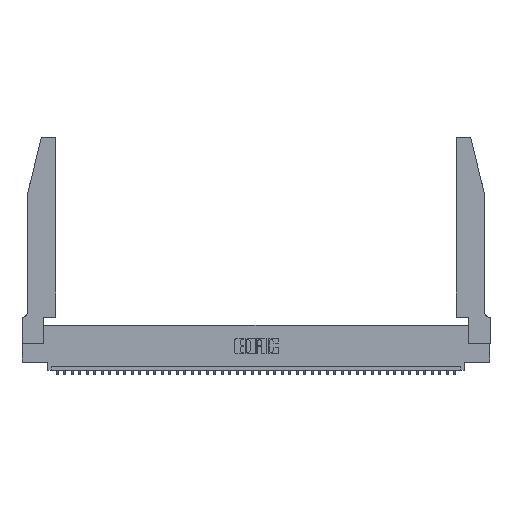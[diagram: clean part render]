
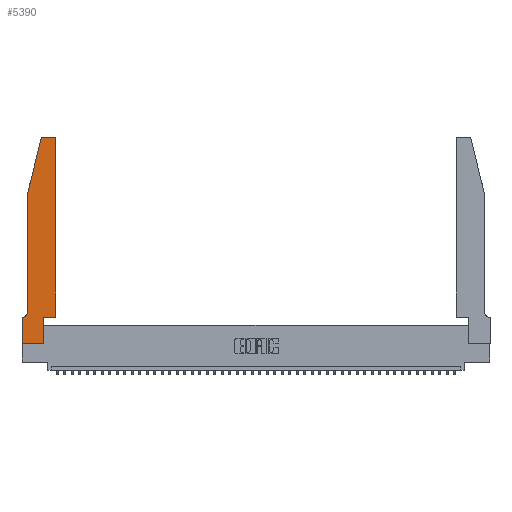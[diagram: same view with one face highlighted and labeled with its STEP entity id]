
A CAD part, top view. The second image highlights one B-rep face of the part: STEP entity #5390.
In plain terms, the highlighted planar face has unit normal (0, 0, 1).
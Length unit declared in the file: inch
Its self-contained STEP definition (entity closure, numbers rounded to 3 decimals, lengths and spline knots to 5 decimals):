
#191 = DIRECTION ( 'NONE',  ( 0., 1., 0. ) ) ;
#806 = VECTOR ( 'NONE', #6028, 39.37008 ) ;
#989 = CARTESIAN_POINT ( 'NONE',  ( 0.2865, 0.35, 0.37 ) ) ;
#1644 = VERTEX_POINT ( 'NONE', #21481 ) ;
#1873 = CARTESIAN_POINT ( 'NONE',  ( 0.0755, 0.42, 0.37 ) ) ;
#1937 = LINE ( 'NONE', #42458, #41774 ) ;
#2378 = ORIENTED_EDGE ( 'NONE', *, *, #20064, .T. ) ;
#2583 = AXIS2_PLACEMENT_3D ( 'NONE', #17825, #21153, #38533 ) ;
#2833 = ORIENTED_EDGE ( 'NONE', *, *, #18375, .T. ) ;
#2907 = EDGE_CURVE ( 'NONE', #39275, #1644, #37408, .T. ) ;
#3115 = LINE ( 'NONE', #5863, #16230 ) ;
#3315 = CARTESIAN_POINT ( 'NONE',  ( 0.2865, 0.35, 0.37 ) ) ;
#3512 = DIRECTION ( 'NONE',  ( 1., 0., 0. ) ) ;
#4232 = AXIS2_PLACEMENT_3D ( 'NONE', #39001, #29052, #32171 ) ;
#4340 = EDGE_CURVE ( 'NONE', #42796, #12998, #38647, .T. ) ;
#4575 = DIRECTION ( 'NONE',  ( 1., 0., 0. ) ) ;
#4819 = ORIENTED_EDGE ( 'NONE', *, *, #34659, .T. ) ;
#5390 = ADVANCED_FACE ( 'NONE', ( #12595 ), #5482, .T. ) ;
#5440 = CARTESIAN_POINT ( 'NONE',  ( 0.4505, 2.72, 0.37 ) ) ;
#5482 = PLANE ( 'NONE',  #21039 ) ;
#5863 = CARTESIAN_POINT ( 'NONE',  ( 0.0755, 2., 0.37 ) ) ;
#6028 = DIRECTION ( 'NONE',  ( 1., 0., 0. ) ) ;
#7231 = VERTEX_POINT ( 'NONE', #1873 ) ;
#7233 = EDGE_LOOP ( 'NONE', ( #24595, #9767, #9809, #29688, #2378, #16241, #39439, #4819, #2833, #15806, #39345, #33789 ) ) ;
#7916 = VERTEX_POINT ( 'NONE', #989 ) ;
#9767 = ORIENTED_EDGE ( 'NONE', *, *, #2907, .T. ) ;
#9809 = ORIENTED_EDGE ( 'NONE', *, *, #25964, .T. ) ;
#10091 = EDGE_CURVE ( 'NONE', #30700, #7231, #3115, .T. ) ;
#11860 = CARTESIAN_POINT ( 'NONE',  ( 0.2605, 2.75, 0.37 ) ) ;
#12595 = FACE_OUTER_BOUND ( 'NONE', #7233, .T. ) ;
#12653 = EDGE_CURVE ( 'NONE', #7916, #32591, #25085, .T. ) ;
#12816 = CIRCLE ( 'NONE', #2583, 0.07 ) ;
#12870 = CARTESIAN_POINT ( 'NONE',  ( 0.4505, 0.35, 0.37 ) ) ;
#12997 = CARTESIAN_POINT ( 'NONE',  ( 0., 0., 0.37 ) ) ;
#12998 = VERTEX_POINT ( 'NONE', #36776 ) ;
#14085 = CARTESIAN_POINT ( 'NONE',  ( 0.0755, 2., 0.37 ) ) ;
#14971 = CARTESIAN_POINT ( 'NONE',  ( 0.4505, 0.35, 0.37 ) ) ;
#15395 = AXIS2_PLACEMENT_3D ( 'NONE', #34845, #24881, #4575 ) ;
#15483 = DIRECTION ( 'NONE',  ( 0., -1., 0. ) ) ;
#15806 = ORIENTED_EDGE ( 'NONE', *, *, #12653, .T. ) ;
#15988 = CARTESIAN_POINT ( 'NONE',  ( 0.0755, 0.35, 0.37 ) ) ;
#16230 = VECTOR ( 'NONE', #26606, 39.37008 ) ;
#16241 = ORIENTED_EDGE ( 'NONE', *, *, #38518, .T. ) ;
#16411 = EDGE_CURVE ( 'NONE', #32591, #42796, #41674, .T. ) ;
#17486 = DIRECTION ( 'NONE',  ( -0.239, -0.971, 0. ) ) ;
#17825 = CARTESIAN_POINT ( 'NONE',  ( 0.0055, 0.42, 0.37 ) ) ;
#18375 = EDGE_CURVE ( 'NONE', #20291, #7916, #23511, .T. ) ;
#19219 = DIRECTION ( 'NONE',  ( -1., 0., 0. ) ) ;
#20064 = EDGE_CURVE ( 'NONE', #7231, #38523, #12816, .T. ) ;
#20291 = VERTEX_POINT ( 'NONE', #29174 ) ;
#20858 = VERTEX_POINT ( 'NONE', #12997 ) ;
#21039 = AXIS2_PLACEMENT_3D ( 'NONE', #33361, #30671, #3512 ) ;
#21153 = DIRECTION ( 'NONE',  ( 0., 0., -1. ) ) ;
#21481 = CARTESIAN_POINT ( 'NONE',  ( 0.25487, 2.72718, 0.37 ) ) ;
#23511 = LINE ( 'NONE', #3315, #27242 ) ;
#24120 = VECTOR ( 'NONE', #42094, 39.37008 ) ;
#24223 = CARTESIAN_POINT ( 'NONE',  ( 0.0755, 2., 0.37 ) ) ;
#24317 = VECTOR ( 'NONE', #17486, 39.37008 ) ;
#24595 = ORIENTED_EDGE ( 'NONE', *, *, #30277, .T. ) ;
#24881 = DIRECTION ( 'NONE',  ( 0., 0., 1. ) ) ;
#25085 = LINE ( 'NONE', #31417, #36790 ) ;
#25964 = EDGE_CURVE ( 'NONE', #1644, #30700, #37609, .T. ) ;
#26606 = DIRECTION ( 'NONE',  ( 0., -1., 0. ) ) ;
#26845 = VERTEX_POINT ( 'NONE', #39020 ) ;
#26910 = EDGE_CURVE ( 'NONE', #26845, #20858, #1937, .T. ) ;
#27242 = VECTOR ( 'NONE', #191, 39.37008 ) ;
#29052 = DIRECTION ( 'NONE',  ( 0., 0., 1. ) ) ;
#29174 = CARTESIAN_POINT ( 'NONE',  ( 0.2865, 0., 0.37 ) ) ;
#29439 = CARTESIAN_POINT ( 'NONE',  ( 0., 0., 0.37 ) ) ;
#29449 = CARTESIAN_POINT ( 'NONE',  ( 0.0055, 0.35, 0.37 ) ) ;
#29688 = ORIENTED_EDGE ( 'NONE', *, *, #10091, .T. ) ;
#29821 = VECTOR ( 'NONE', #19219, 39.37008 ) ;
#30277 = EDGE_CURVE ( 'NONE', #12998, #39275, #42588, .T. ) ;
#30671 = DIRECTION ( 'NONE',  ( 0., 0., 1. ) ) ;
#30700 = VERTEX_POINT ( 'NONE', #24223 ) ;
#31417 = CARTESIAN_POINT ( 'NONE',  ( 0.4505, 0.35, 0.37 ) ) ;
#32171 = DIRECTION ( 'NONE',  ( 1., 0., 0. ) ) ;
#32535 = VECTOR ( 'NONE', #39118, 39.37008 ) ;
#32591 = VERTEX_POINT ( 'NONE', #12870 ) ;
#33361 = CARTESIAN_POINT ( 'NONE',  ( 0., 0.35, 0.37 ) ) ;
#33789 = ORIENTED_EDGE ( 'NONE', *, *, #4340, .T. ) ;
#34286 = CARTESIAN_POINT ( 'NONE',  ( 0.284, 2.75, 0.37 ) ) ;
#34659 = EDGE_CURVE ( 'NONE', #20858, #20291, #42230, .T. ) ;
#34845 = CARTESIAN_POINT ( 'NONE',  ( 0.4205, 2.72, 0.37 ) ) ;
#35641 = LINE ( 'NONE', #15988, #29821 ) ;
#36776 = CARTESIAN_POINT ( 'NONE',  ( 0.4205, 2.75, 0.37 ) ) ;
#36790 = VECTOR ( 'NONE', #41830, 39.37008 ) ;
#37408 = CIRCLE ( 'NONE', #4232, 0.03 ) ;
#37609 = LINE ( 'NONE', #14085, #24317 ) ;
#38518 = EDGE_CURVE ( 'NONE', #38523, #26845, #35641, .T. ) ;
#38523 = VERTEX_POINT ( 'NONE', #29449 ) ;
#38533 = DIRECTION ( 'NONE',  ( -1., 0., 0. ) ) ;
#38647 = CIRCLE ( 'NONE', #15395, 0.03 ) ;
#39001 = CARTESIAN_POINT ( 'NONE',  ( 0.284, 2.72, 0.37 ) ) ;
#39020 = CARTESIAN_POINT ( 'NONE',  ( 0., 0.35, 0.37 ) ) ;
#39118 = DIRECTION ( 'NONE',  ( -1., 0., 0. ) ) ;
#39275 = VERTEX_POINT ( 'NONE', #34286 ) ;
#39345 = ORIENTED_EDGE ( 'NONE', *, *, #16411, .T. ) ;
#39439 = ORIENTED_EDGE ( 'NONE', *, *, #26910, .T. ) ;
#41674 = LINE ( 'NONE', #14971, #24120 ) ;
#41774 = VECTOR ( 'NONE', #15483, 39.37008 ) ;
#41830 = DIRECTION ( 'NONE',  ( 1., 0., 0. ) ) ;
#42094 = DIRECTION ( 'NONE',  ( 0., 1., 0. ) ) ;
#42230 = LINE ( 'NONE', #29439, #806 ) ;
#42458 = CARTESIAN_POINT ( 'NONE',  ( 0., 0., 0.37 ) ) ;
#42588 = LINE ( 'NONE', #11860, #32535 ) ;
#42796 = VERTEX_POINT ( 'NONE', #5440 ) ;
